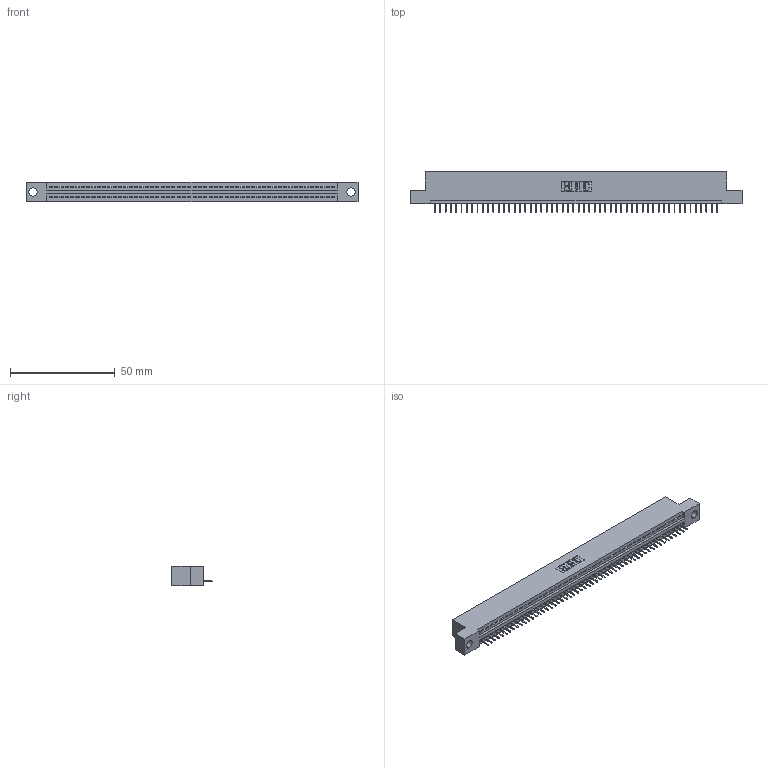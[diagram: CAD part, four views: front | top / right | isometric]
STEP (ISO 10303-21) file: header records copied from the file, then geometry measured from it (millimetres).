
FILE_DESCRIPTION (( 'STEP AP203' ), '1' );
FILE_NAME ('395-054-524-104.STEP', '2021-05-31T21:33:09', ( '' ), ( '' ), 'SwSTEP 2.0', 'SolidWorks 2020', '' );
FILE_SCHEMA (( 'CONFIG_CONTROL_DESIGN' ));
Length unit declared in the file: inch
Products named in the file (3): 345-292-001_345-293-124; 395-054-524-104; 345 Part_Flush Mounting Lugs - 0.156 Dia-TI
Assembly tree (55 placements, depth 2):
  395-054-524-104
    345 Part_Flush Mounting Lugs - 0.156 Dia-TI
    345-292-001_345-293-124  x54
Bounding box: 158.37 x 19.35 x 9.4 mm (x, y, z)
Volume: 14821.1 mm3; surface area: 19019.4 mm2
Topology: 55 solids, 55 shells, 3488 faces, 10097 edges, 6514 vertices
Faces by surface type: plane 2578, cylinder 910
Entity records: 39519 total; most frequent: CARTESIAN_POINT 6852, ORIENTED_EDGE 6838, DIRECTION 5967, EDGE_CURVE 3419, VECTOR 3075, LINE 3075, VERTEX_POINT 2274, AXIS2_PLACEMENT_3D 1446
